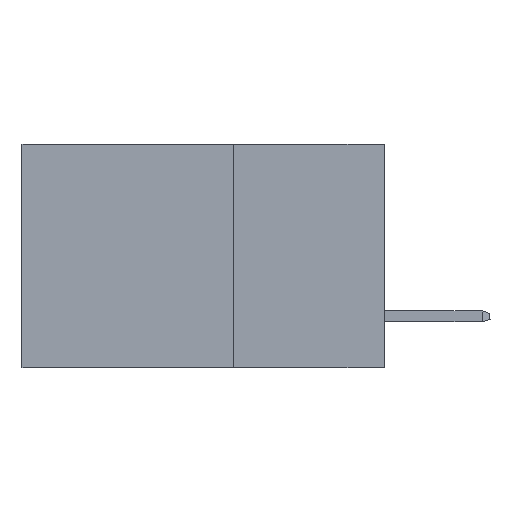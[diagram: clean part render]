
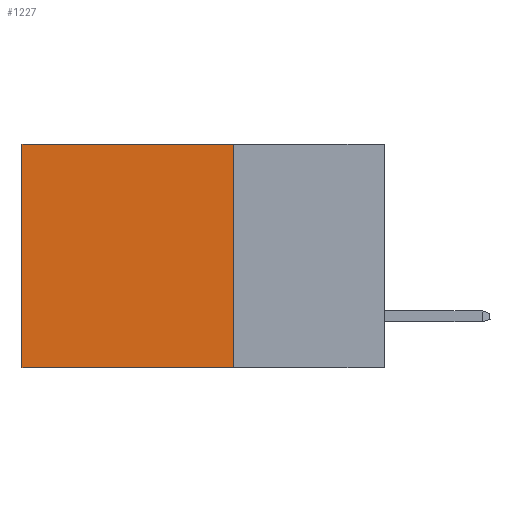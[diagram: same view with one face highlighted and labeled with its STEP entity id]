
A CAD part, left-side view. The second image highlights one B-rep face of the part: STEP entity #1227.
In plain terms, the highlighted planar face has unit normal (-1, 0, 0).
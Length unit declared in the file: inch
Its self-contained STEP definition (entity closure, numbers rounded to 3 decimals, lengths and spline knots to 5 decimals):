
#397 = EDGE_CURVE ( 'NONE', #13794, #7164, #12416, .T. ) ;
#1227 = ADVANCED_FACE ( 'NONE', ( #6896 ), #10352, .F. ) ;
#1417 = LINE ( 'NONE', #2099, #5334 ) ;
#1458 = CARTESIAN_POINT ( 'NONE',  ( 0.2615, 0.6, -0.37 ) ) ;
#1755 = EDGE_CURVE ( 'NONE', #13794, #11853, #1417, .T. ) ;
#2099 = CARTESIAN_POINT ( 'NONE',  ( 0.2615, 0.25, -0.37 ) ) ;
#2722 = VECTOR ( 'NONE', #5749, 39.37008 ) ;
#3339 = DIRECTION ( 'NONE',  ( 0., 0., -1. ) ) ;
#3678 = CARTESIAN_POINT ( 'NONE',  ( 0.2615, 0.6, -0.37 ) ) ;
#3810 = CARTESIAN_POINT ( 'NONE',  ( 0.2615, 0.25, -0.37 ) ) ;
#4754 = DIRECTION ( 'NONE',  ( 0., 1., 0. ) ) ;
#5004 = CARTESIAN_POINT ( 'NONE',  ( 0.2615, 0.25, -0.37 ) ) ;
#5334 = VECTOR ( 'NONE', #3339, 39.37008 ) ;
#5749 = DIRECTION ( 'NONE',  ( 0., 0., -1. ) ) ;
#5946 = DIRECTION ( 'NONE',  ( 0., 0., -1. ) ) ;
#6394 = VECTOR ( 'NONE', #10268, 39.37008 ) ;
#6415 = AXIS2_PLACEMENT_3D ( 'NONE', #3810, #11461, #5946 ) ;
#6765 = VERTEX_POINT ( 'NONE', #3678 ) ;
#6896 = FACE_OUTER_BOUND ( 'NONE', #9415, .T. ) ;
#6984 = CARTESIAN_POINT ( 'NONE',  ( 0.2615, 0.25, 0. ) ) ;
#7164 = VERTEX_POINT ( 'NONE', #13271 ) ;
#7475 = LINE ( 'NONE', #11324, #13664 ) ;
#7555 = EDGE_CURVE ( 'NONE', #11853, #6765, #7475, .T. ) ;
#7822 = ORIENTED_EDGE ( 'NONE', *, *, #397, .T. ) ;
#7966 = ORIENTED_EDGE ( 'NONE', *, *, #7555, .F. ) ;
#8256 = EDGE_CURVE ( 'NONE', #7164, #6765, #12954, .T. ) ;
#9415 = EDGE_LOOP ( 'NONE', ( #9535, #7966, #13775, #7822 ) ) ;
#9535 = ORIENTED_EDGE ( 'NONE', *, *, #8256, .T. ) ;
#9926 = CARTESIAN_POINT ( 'NONE',  ( 0.2615, 0.25, 0. ) ) ;
#10268 = DIRECTION ( 'NONE',  ( 0., 1., 0. ) ) ;
#10352 = PLANE ( 'NONE',  #6415 ) ;
#11324 = CARTESIAN_POINT ( 'NONE',  ( 0.2615, 0.25, -0.37 ) ) ;
#11461 = DIRECTION ( 'NONE',  ( 1., 0., 0. ) ) ;
#11853 = VERTEX_POINT ( 'NONE', #5004 ) ;
#12416 = LINE ( 'NONE', #6984, #6394 ) ;
#12954 = LINE ( 'NONE', #1458, #2722 ) ;
#13271 = CARTESIAN_POINT ( 'NONE',  ( 0.2615, 0.6, 0. ) ) ;
#13664 = VECTOR ( 'NONE', #4754, 39.37008 ) ;
#13775 = ORIENTED_EDGE ( 'NONE', *, *, #1755, .F. ) ;
#13794 = VERTEX_POINT ( 'NONE', #9926 ) ;
